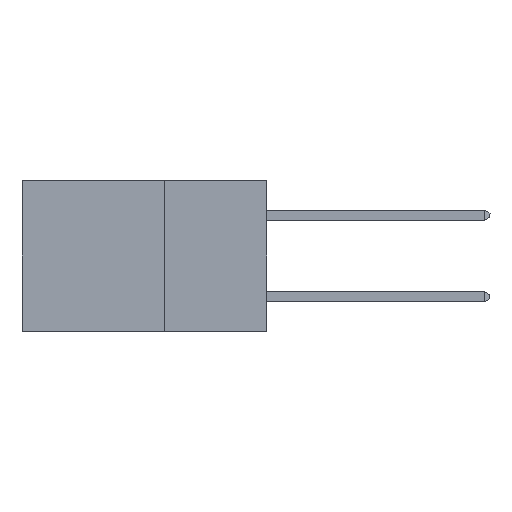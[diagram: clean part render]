
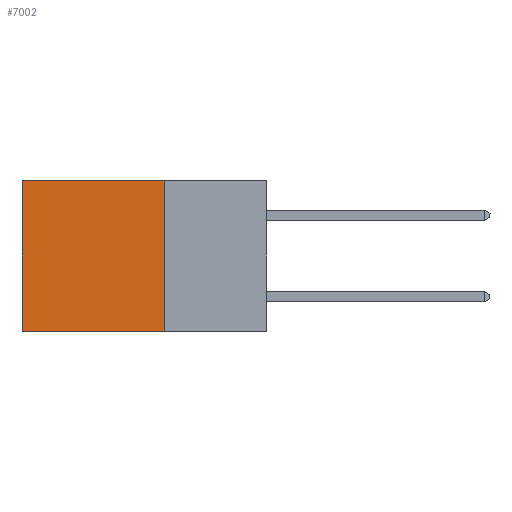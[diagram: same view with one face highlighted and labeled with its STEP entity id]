
A CAD part, left-side view. The second image highlights one B-rep face of the part: STEP entity #7002.
In plain terms, the highlighted planar face has unit normal (-1, 0, 0).
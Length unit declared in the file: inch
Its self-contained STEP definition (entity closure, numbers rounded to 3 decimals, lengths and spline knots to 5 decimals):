
#104 = CARTESIAN_POINT ( 'NONE',  ( 0.2875, 0.25, -0.37 ) ) ;
#159 = PLANE ( 'NONE',  #10191 ) ;
#987 = CARTESIAN_POINT ( 'NONE',  ( 0.2875, 0.6, 0. ) ) ;
#2272 = LINE ( 'NONE', #5220, #8899 ) ;
#2407 = EDGE_CURVE ( 'NONE', #10670, #10042, #14858, .T. ) ;
#2864 = DIRECTION ( 'NONE',  ( 0., 1., 0. ) ) ;
#3663 = CARTESIAN_POINT ( 'NONE',  ( 0.2875, 0.25, 0. ) ) ;
#3741 = EDGE_LOOP ( 'NONE', ( #6762, #6814, #7081, #7095 ) ) ;
#4011 = DIRECTION ( 'NONE',  ( 1., 0., 0. ) ) ;
#5220 = CARTESIAN_POINT ( 'NONE',  ( 0.2875, 0.6, 0. ) ) ;
#5311 = EDGE_CURVE ( 'NONE', #14166, #8706, #15685, .T. ) ;
#5830 = EDGE_CURVE ( 'NONE', #8706, #10042, #2272, .T. ) ;
#6762 = ORIENTED_EDGE ( 'NONE', *, *, #5830, .T. ) ;
#6814 = ORIENTED_EDGE ( 'NONE', *, *, #2407, .F. ) ;
#7002 = ADVANCED_FACE ( 'NONE', ( #9676 ), #159, .F. ) ;
#7081 = ORIENTED_EDGE ( 'NONE', *, *, #9558, .F. ) ;
#7095 = ORIENTED_EDGE ( 'NONE', *, *, #5311, .T. ) ;
#7711 = DIRECTION ( 'NONE',  ( 0., 0., -1. ) ) ;
#7864 = DIRECTION ( 'NONE',  ( 0., 1., 0. ) ) ;
#8102 = CARTESIAN_POINT ( 'NONE',  ( 0.2875, 0.25, 0. ) ) ;
#8518 = LINE ( 'NONE', #8102, #14579 ) ;
#8706 = VERTEX_POINT ( 'NONE', #987 ) ;
#8899 = VECTOR ( 'NONE', #7711, 39.37008 ) ;
#9336 = VECTOR ( 'NONE', #7864, 39.37008 ) ;
#9558 = EDGE_CURVE ( 'NONE', #14166, #10670, #8518, .T. ) ;
#9676 = FACE_OUTER_BOUND ( 'NONE', #3741, .T. ) ;
#10042 = VERTEX_POINT ( 'NONE', #13851 ) ;
#10191 = AXIS2_PLACEMENT_3D ( 'NONE', #11486, #4011, #12696 ) ;
#10670 = VERTEX_POINT ( 'NONE', #104 ) ;
#11486 = CARTESIAN_POINT ( 'NONE',  ( 0.2875, 0.25, 0. ) ) ;
#11732 = VECTOR ( 'NONE', #2864, 39.37008 ) ;
#11837 = DIRECTION ( 'NONE',  ( 0., 0., -1. ) ) ;
#12696 = DIRECTION ( 'NONE',  ( 0., 0., -1. ) ) ;
#12765 = CARTESIAN_POINT ( 'NONE',  ( 0.2875, 0.25, 0. ) ) ;
#13080 = CARTESIAN_POINT ( 'NONE',  ( 0.2875, 0.25, -0.37 ) ) ;
#13851 = CARTESIAN_POINT ( 'NONE',  ( 0.2875, 0.6, -0.37 ) ) ;
#14166 = VERTEX_POINT ( 'NONE', #3663 ) ;
#14579 = VECTOR ( 'NONE', #11837, 39.37008 ) ;
#14858 = LINE ( 'NONE', #13080, #11732 ) ;
#15685 = LINE ( 'NONE', #12765, #9336 ) ;
